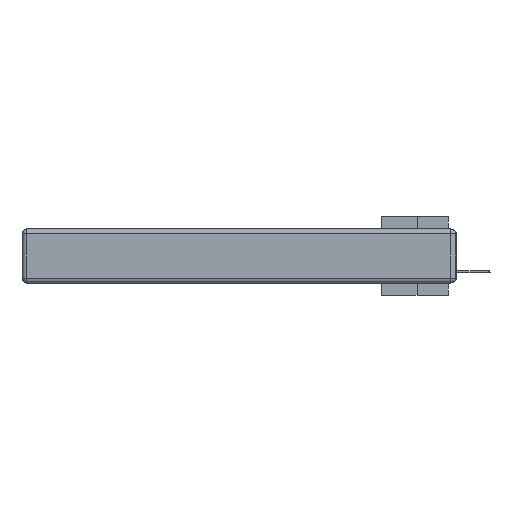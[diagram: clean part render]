
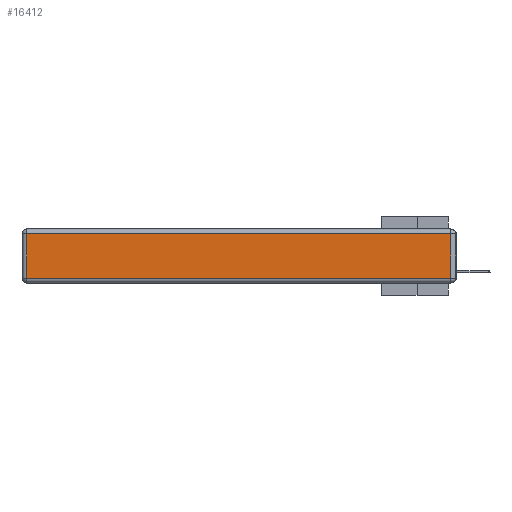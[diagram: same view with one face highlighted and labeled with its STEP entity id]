
A CAD part, left-side view. The second image highlights one B-rep face of the part: STEP entity #16412.
In plain terms, the highlighted planar face has unit normal (-1, 0, 0).
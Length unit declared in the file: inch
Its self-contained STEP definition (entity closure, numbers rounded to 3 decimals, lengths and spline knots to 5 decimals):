
#268 = EDGE_LOOP ( 'NONE', ( #13628, #11667, #18200, #22723 ) ) ;
#305 = VERTEX_POINT ( 'NONE', #6711 ) ;
#568 = DIRECTION ( 'NONE',  ( 0., 1., 0. ) ) ;
#1458 = EDGE_CURVE ( 'NONE', #6864, #7142, #12438, .T. ) ;
#2196 = PLANE ( 'NONE',  #11309 ) ;
#4107 = LINE ( 'NONE', #6578, #28799 ) ;
#4779 = LINE ( 'NONE', #10510, #16065 ) ;
#6017 = EDGE_CURVE ( 'NONE', #305, #18054, #17529, .T. ) ;
#6028 = CARTESIAN_POINT ( 'NONE',  ( 0., 2.72, -0.313 ) ) ;
#6578 = CARTESIAN_POINT ( 'NONE',  ( 0., 2.72, -0.343 ) ) ;
#6711 = CARTESIAN_POINT ( 'NONE',  ( 0., 0.03, -0.03 ) ) ;
#6819 = DIRECTION ( 'NONE',  ( 0., -1., 0. ) ) ;
#6864 = VERTEX_POINT ( 'NONE', #6028 ) ;
#6990 = VECTOR ( 'NONE', #568, 39.37008 ) ;
#7068 = FACE_OUTER_BOUND ( 'NONE', #268, .T. ) ;
#7142 = VERTEX_POINT ( 'NONE', #24996 ) ;
#7515 = EDGE_CURVE ( 'NONE', #7142, #305, #4779, .T. ) ;
#10510 = CARTESIAN_POINT ( 'NONE',  ( 0., 0.03, -0.343 ) ) ;
#11309 = AXIS2_PLACEMENT_3D ( 'NONE', #20194, #15369, #29174 ) ;
#11667 = ORIENTED_EDGE ( 'NONE', *, *, #7515, .T. ) ;
#12438 = LINE ( 'NONE', #15693, #17691 ) ;
#12864 = EDGE_CURVE ( 'NONE', #18054, #6864, #4107, .T. ) ;
#13628 = ORIENTED_EDGE ( 'NONE', *, *, #1458, .T. ) ;
#14017 = CARTESIAN_POINT ( 'NONE',  ( 0., 2.75, -0.03 ) ) ;
#15369 = DIRECTION ( 'NONE',  ( -1., 0., 0. ) ) ;
#15693 = CARTESIAN_POINT ( 'NONE',  ( 0., 0., -0.313 ) ) ;
#16065 = VECTOR ( 'NONE', #17481, 39.37008 ) ;
#16412 = ADVANCED_FACE ( 'NONE', ( #7068 ), #2196, .T. ) ;
#17025 = CARTESIAN_POINT ( 'NONE',  ( 0., 2.72, -0.03 ) ) ;
#17481 = DIRECTION ( 'NONE',  ( 0., 0., 1. ) ) ;
#17529 = LINE ( 'NONE', #14017, #6990 ) ;
#17691 = VECTOR ( 'NONE', #6819, 39.37008 ) ;
#18054 = VERTEX_POINT ( 'NONE', #17025 ) ;
#18200 = ORIENTED_EDGE ( 'NONE', *, *, #6017, .T. ) ;
#20162 = DIRECTION ( 'NONE',  ( 0., 0., -1. ) ) ;
#20194 = CARTESIAN_POINT ( 'NONE',  ( 0., 0., -0.343 ) ) ;
#22723 = ORIENTED_EDGE ( 'NONE', *, *, #12864, .T. ) ;
#24996 = CARTESIAN_POINT ( 'NONE',  ( 0., 0.03, -0.313 ) ) ;
#28799 = VECTOR ( 'NONE', #20162, 39.37008 ) ;
#29174 = DIRECTION ( 'NONE',  ( 0., 0., 1. ) ) ;
